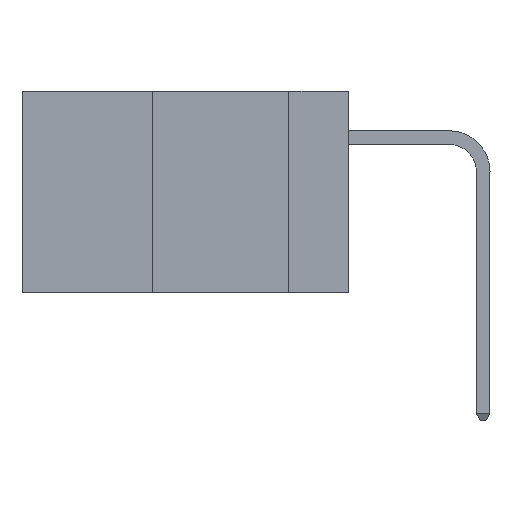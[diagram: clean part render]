
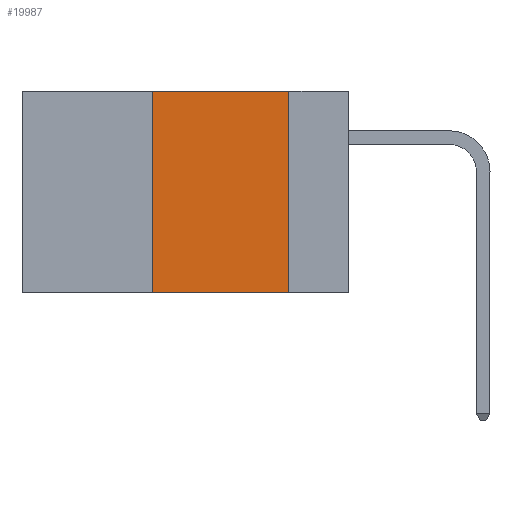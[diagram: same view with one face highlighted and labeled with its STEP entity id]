
A CAD part, left-side view. The second image highlights one B-rep face of the part: STEP entity #19987.
In plain terms, the highlighted planar face has unit normal (-1, 0, 0).
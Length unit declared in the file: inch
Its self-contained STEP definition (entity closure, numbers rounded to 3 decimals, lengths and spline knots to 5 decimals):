
#357 = DIRECTION ( 'NONE',  ( 0., -1., 0. ) ) ;
#1021 = CARTESIAN_POINT ( 'NONE',  ( 0., 0.36, -0.37 ) ) ;
#1279 = LINE ( 'NONE', #23266, #16024 ) ;
#2061 = EDGE_CURVE ( 'NONE', #33930, #26385, #7070, .T. ) ;
#2499 = DIRECTION ( 'NONE',  ( 0., 0., 1. ) ) ;
#2871 = CARTESIAN_POINT ( 'NONE',  ( 0., 0.6, 0. ) ) ;
#3638 = CARTESIAN_POINT ( 'NONE',  ( 0., 0.36, 0. ) ) ;
#5582 = VECTOR ( 'NONE', #15299, 39.37008 ) ;
#6438 = CARTESIAN_POINT ( 'NONE',  ( 0., 0.6, -0.37 ) ) ;
#7062 = ORIENTED_EDGE ( 'NONE', *, *, #11958, .T. ) ;
#7070 = LINE ( 'NONE', #34533, #21843 ) ;
#11538 = LINE ( 'NONE', #6438, #21233 ) ;
#11754 = DIRECTION ( 'NONE',  ( 1., 0., 0. ) ) ;
#11958 = EDGE_CURVE ( 'NONE', #33930, #18161, #11538, .T. ) ;
#12511 = VERTEX_POINT ( 'NONE', #32471 ) ;
#14320 = LINE ( 'NONE', #35614, #5582 ) ;
#15299 = DIRECTION ( 'NONE',  ( 0., 0., -1. ) ) ;
#16024 = VECTOR ( 'NONE', #37681, 39.37008 ) ;
#18161 = VERTEX_POINT ( 'NONE', #23490 ) ;
#19987 = ADVANCED_FACE ( 'NONE', ( #22077 ), #29297, .F. ) ;
#21233 = VECTOR ( 'NONE', #357, 39.37008 ) ;
#21713 = ORIENTED_EDGE ( 'NONE', *, *, #27533, .F. ) ;
#21838 = ORIENTED_EDGE ( 'NONE', *, *, #32238, .F. ) ;
#21843 = VECTOR ( 'NONE', #2499, 39.37008 ) ;
#22077 = FACE_OUTER_BOUND ( 'NONE', #28937, .T. ) ;
#22981 = ORIENTED_EDGE ( 'NONE', *, *, #2061, .F. ) ;
#23266 = CARTESIAN_POINT ( 'NONE',  ( 0., 0.6, 0. ) ) ;
#23490 = CARTESIAN_POINT ( 'NONE',  ( 0., 0.11, -0.37 ) ) ;
#26385 = VERTEX_POINT ( 'NONE', #3638 ) ;
#26657 = AXIS2_PLACEMENT_3D ( 'NONE', #2871, #11754, #32159 ) ;
#27533 = EDGE_CURVE ( 'NONE', #26385, #12511, #1279, .T. ) ;
#28937 = EDGE_LOOP ( 'NONE', ( #21838, #21713, #22981, #7062 ) ) ;
#29297 = PLANE ( 'NONE',  #26657 ) ;
#32159 = DIRECTION ( 'NONE',  ( 0., 0., -1. ) ) ;
#32238 = EDGE_CURVE ( 'NONE', #12511, #18161, #14320, .T. ) ;
#32471 = CARTESIAN_POINT ( 'NONE',  ( 0., 0.11, 0. ) ) ;
#33930 = VERTEX_POINT ( 'NONE', #1021 ) ;
#34533 = CARTESIAN_POINT ( 'NONE',  ( 0., 0.36, 0. ) ) ;
#35614 = CARTESIAN_POINT ( 'NONE',  ( 0., 0.11, 0. ) ) ;
#37681 = DIRECTION ( 'NONE',  ( 0., -1., 0. ) ) ;
